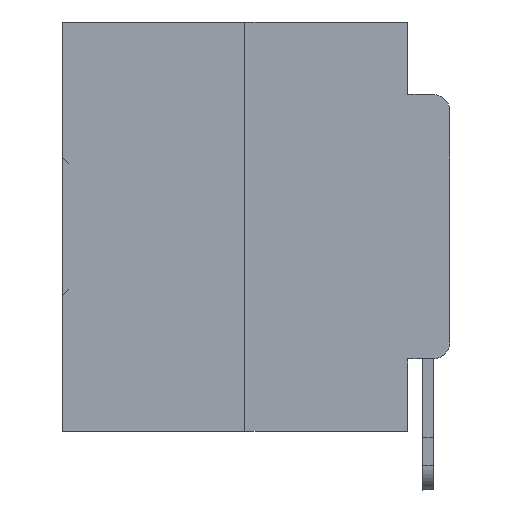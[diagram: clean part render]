
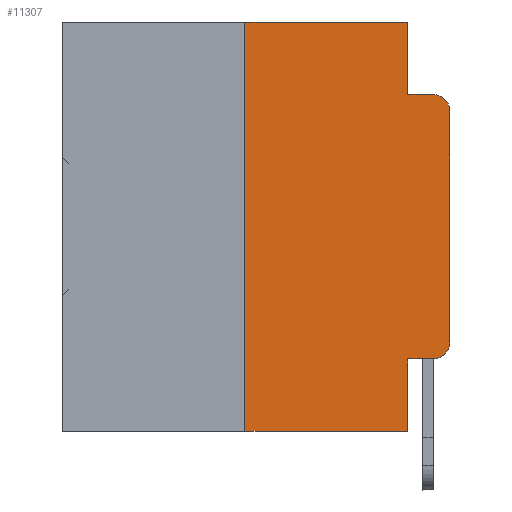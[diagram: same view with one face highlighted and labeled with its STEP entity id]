
A CAD part, left-side view. The second image highlights one B-rep face of the part: STEP entity #11307.
In plain terms, the highlighted planar face has unit normal (-1, 0, 0).
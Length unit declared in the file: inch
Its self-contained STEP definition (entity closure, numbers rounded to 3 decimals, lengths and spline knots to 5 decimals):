
#929 = EDGE_CURVE ( 'NONE', #33924, #4664, #16352, .T. ) ;
#1870 = CARTESIAN_POINT ( 'NONE',  ( 0., 0.051, -0.4115 ) ) ;
#2621 = ORIENTED_EDGE ( 'NONE', *, *, #2701, .T. ) ;
#2701 = EDGE_CURVE ( 'NONE', #10190, #28016, #4080, .T. ) ;
#2986 = DIRECTION ( 'NONE',  ( 0., 0., -1. ) ) ;
#4080 = LINE ( 'NONE', #30142, #28306 ) ;
#4194 = LINE ( 'NONE', #11055, #31917 ) ;
#4240 = VECTOR ( 'NONE', #7507, 39.37008 ) ;
#4664 = VERTEX_POINT ( 'NONE', #30414 ) ;
#4673 = LINE ( 'NONE', #27752, #28935 ) ;
#5129 = CARTESIAN_POINT ( 'NONE',  ( 0., 0., -0.1085 ) ) ;
#5639 = CARTESIAN_POINT ( 'NONE',  ( 0., 0.25, 0. ) ) ;
#5911 = VERTEX_POINT ( 'NONE', #5639 ) ;
#5931 = VECTOR ( 'NONE', #33732, 39.37008 ) ;
#5944 = VECTOR ( 'NONE', #11440, 39.37008 ) ;
#6208 = ORIENTED_EDGE ( 'NONE', *, *, #20626, .T. ) ;
#6705 = VERTEX_POINT ( 'NONE', #33879 ) ;
#7310 = EDGE_CURVE ( 'NONE', #15495, #26868, #4673, .T. ) ;
#7507 = DIRECTION ( 'NONE',  ( 0., -1., 0. ) ) ;
#7527 = CARTESIAN_POINT ( 'NONE',  ( 0., 0.02, -0.0885 ) ) ;
#7911 = ORIENTED_EDGE ( 'NONE', *, *, #22315, .F. ) ;
#8276 = CARTESIAN_POINT ( 'NONE',  ( 0., 0., -0.3915 ) ) ;
#10190 = VERTEX_POINT ( 'NONE', #8276 ) ;
#10289 = DIRECTION ( 'NONE',  ( 0., 0., -1. ) ) ;
#10468 = AXIS2_PLACEMENT_3D ( 'NONE', #26767, #23894, #10289 ) ;
#10775 = CARTESIAN_POINT ( 'NONE',  ( 0., 0.473, 0. ) ) ;
#11055 = CARTESIAN_POINT ( 'NONE',  ( 0., 0.25, 0. ) ) ;
#11307 = ADVANCED_FACE ( 'NONE', ( #32147 ), #35687, .F. ) ;
#11323 = CARTESIAN_POINT ( 'NONE',  ( 0., 0.051, 0. ) ) ;
#11380 = LINE ( 'NONE', #29773, #28712 ) ;
#11440 = DIRECTION ( 'NONE',  ( 0., 0., -1. ) ) ;
#11552 = ORIENTED_EDGE ( 'NONE', *, *, #7310, .F. ) ;
#11778 = ORIENTED_EDGE ( 'NONE', *, *, #33513, .F. ) ;
#13178 = DIRECTION ( 'NONE',  ( 0., 0., -1. ) ) ;
#13326 = LINE ( 'NONE', #11323, #5944 ) ;
#13577 = VECTOR ( 'NONE', #35535, 39.37008 ) ;
#13616 = LINE ( 'NONE', #1870, #13577 ) ;
#13765 = CARTESIAN_POINT ( 'NONE',  ( 0., 0.051, -0.0885 ) ) ;
#15169 = CARTESIAN_POINT ( 'NONE',  ( 0., 0.051, 0. ) ) ;
#15495 = VERTEX_POINT ( 'NONE', #13765 ) ;
#16352 = LINE ( 'NONE', #20093, #5931 ) ;
#16574 = DIRECTION ( 'NONE',  ( 1., 0., 0. ) ) ;
#16856 = AXIS2_PLACEMENT_3D ( 'NONE', #27569, #19835, #2986 ) ;
#17228 = LINE ( 'NONE', #18686, #4240 ) ;
#17312 = VERTEX_POINT ( 'NONE', #15169 ) ;
#17721 = AXIS2_PLACEMENT_3D ( 'NONE', #10775, #16574, #35933 ) ;
#18686 = CARTESIAN_POINT ( 'NONE',  ( 0., 0.473, 0. ) ) ;
#18877 = ORIENTED_EDGE ( 'NONE', *, *, #24564, .T. ) ;
#18906 = CARTESIAN_POINT ( 'NONE',  ( 0., 0.25, -0.5 ) ) ;
#19707 = EDGE_CURVE ( 'NONE', #17312, #15495, #13326, .T. ) ;
#19835 = DIRECTION ( 'NONE',  ( -1., 0., 0. ) ) ;
#20044 = EDGE_CURVE ( 'NONE', #5911, #17312, #17228, .T. ) ;
#20093 = CARTESIAN_POINT ( 'NONE',  ( 0., 0.473, -0.5 ) ) ;
#20626 = EDGE_CURVE ( 'NONE', #26817, #10190, #31451, .T. ) ;
#22315 = EDGE_CURVE ( 'NONE', #6705, #4664, #11380, .T. ) ;
#23112 = ORIENTED_EDGE ( 'NONE', *, *, #929, .T. ) ;
#23894 = DIRECTION ( 'NONE',  ( -1., 0., 0. ) ) ;
#24537 = DIRECTION ( 'NONE',  ( 0., 0., 1. ) ) ;
#24564 = EDGE_CURVE ( 'NONE', #28016, #26868, #34894, .T. ) ;
#24688 = EDGE_LOOP ( 'NONE', ( #2621, #18877, #11552, #32444, #33053, #11778, #23112, #7911, #31699, #6208 ) ) ;
#26420 = EDGE_CURVE ( 'NONE', #6705, #26817, #13616, .T. ) ;
#26767 = CARTESIAN_POINT ( 'NONE',  ( 0., 0.02, -0.3915 ) ) ;
#26817 = VERTEX_POINT ( 'NONE', #34912 ) ;
#26868 = VERTEX_POINT ( 'NONE', #7527 ) ;
#27569 = CARTESIAN_POINT ( 'NONE',  ( 0., 0.02, -0.1085 ) ) ;
#27752 = CARTESIAN_POINT ( 'NONE',  ( 0., 0.051, -0.0885 ) ) ;
#28016 = VERTEX_POINT ( 'NONE', #5129 ) ;
#28306 = VECTOR ( 'NONE', #33006, 39.37008 ) ;
#28712 = VECTOR ( 'NONE', #13178, 39.37008 ) ;
#28935 = VECTOR ( 'NONE', #30434, 39.37008 ) ;
#29773 = CARTESIAN_POINT ( 'NONE',  ( 0., 0.051, 0. ) ) ;
#30142 = CARTESIAN_POINT ( 'NONE',  ( 0., 0., 0. ) ) ;
#30414 = CARTESIAN_POINT ( 'NONE',  ( 0., 0.051, -0.5 ) ) ;
#30434 = DIRECTION ( 'NONE',  ( 0., -1., 0. ) ) ;
#31451 = CIRCLE ( 'NONE', #10468, 0.02 ) ;
#31699 = ORIENTED_EDGE ( 'NONE', *, *, #26420, .T. ) ;
#31917 = VECTOR ( 'NONE', #24537, 39.37008 ) ;
#32147 = FACE_OUTER_BOUND ( 'NONE', #24688, .T. ) ;
#32444 = ORIENTED_EDGE ( 'NONE', *, *, #19707, .F. ) ;
#33006 = DIRECTION ( 'NONE',  ( 0., 0., 1. ) ) ;
#33053 = ORIENTED_EDGE ( 'NONE', *, *, #20044, .F. ) ;
#33513 = EDGE_CURVE ( 'NONE', #33924, #5911, #4194, .T. ) ;
#33732 = DIRECTION ( 'NONE',  ( 0., -1., 0. ) ) ;
#33879 = CARTESIAN_POINT ( 'NONE',  ( 0., 0.051, -0.4115 ) ) ;
#33924 = VERTEX_POINT ( 'NONE', #18906 ) ;
#34894 = CIRCLE ( 'NONE', #16856, 0.02 ) ;
#34912 = CARTESIAN_POINT ( 'NONE',  ( 0., 0.02, -0.4115 ) ) ;
#35535 = DIRECTION ( 'NONE',  ( 0., -1., 0. ) ) ;
#35687 = PLANE ( 'NONE',  #17721 ) ;
#35933 = DIRECTION ( 'NONE',  ( 0., 0., -1. ) ) ;
